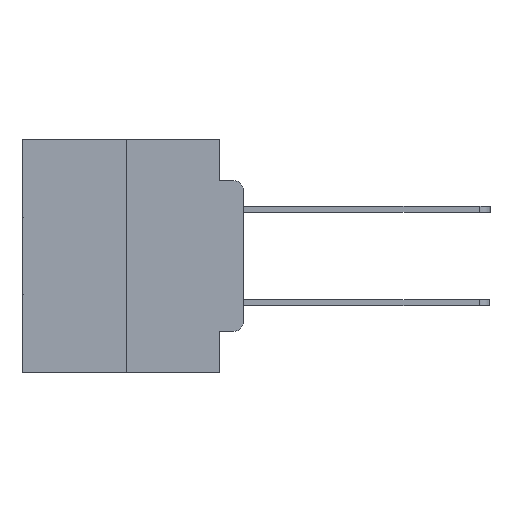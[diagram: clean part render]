
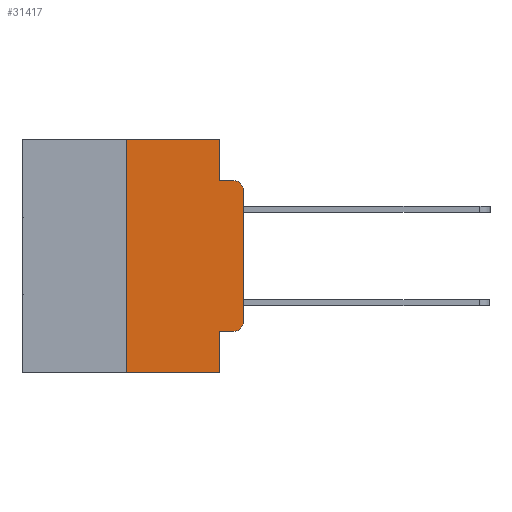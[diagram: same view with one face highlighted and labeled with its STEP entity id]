
A CAD part, left-side view. The second image highlights one B-rep face of the part: STEP entity #31417.
In plain terms, the highlighted planar face has unit normal (-1, 0, 0).
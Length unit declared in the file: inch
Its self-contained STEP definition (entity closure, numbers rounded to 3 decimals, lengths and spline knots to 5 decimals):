
#404 = VERTEX_POINT ( 'NONE', #24986 ) ;
#2196 = DIRECTION ( 'NONE',  ( -1., 0., 0. ) ) ;
#2727 = CARTESIAN_POINT ( 'NONE',  ( 0., 0.051, -0.5 ) ) ;
#2791 = ORIENTED_EDGE ( 'NONE', *, *, #20344, .T. ) ;
#3180 = CARTESIAN_POINT ( 'NONE',  ( 0., 0.02, -0.1085 ) ) ;
#3460 = DIRECTION ( 'NONE',  ( 0., 0., -1. ) ) ;
#4398 = CARTESIAN_POINT ( 'NONE',  ( 0., 0.051, -0.4115 ) ) ;
#4464 = VECTOR ( 'NONE', #26174, 39.37008 ) ;
#4697 = CARTESIAN_POINT ( 'NONE',  ( 0., 0., 0. ) ) ;
#5798 = DIRECTION ( 'NONE',  ( 0., 0., -1. ) ) ;
#6577 = LINE ( 'NONE', #20827, #12320 ) ;
#6727 = EDGE_CURVE ( 'NONE', #28806, #22925, #30735, .T. ) ;
#6857 = DIRECTION ( 'NONE',  ( 0., 0., -1. ) ) ;
#6976 = VERTEX_POINT ( 'NONE', #17495 ) ;
#7261 = CARTESIAN_POINT ( 'NONE',  ( 0., 0., -0.3915 ) ) ;
#7346 = EDGE_CURVE ( 'NONE', #23276, #28806, #10422, .T. ) ;
#7831 = DIRECTION ( 'NONE',  ( 0., -1., 0. ) ) ;
#8003 = ORIENTED_EDGE ( 'NONE', *, *, #7346, .F. ) ;
#8252 = ORIENTED_EDGE ( 'NONE', *, *, #17773, .T. ) ;
#8449 = PLANE ( 'NONE',  #17743 ) ;
#9687 = DIRECTION ( 'NONE',  ( 0., 0., 1. ) ) ;
#9902 = CARTESIAN_POINT ( 'NONE',  ( 0., 0.051, -0.0885 ) ) ;
#10422 = LINE ( 'NONE', #25810, #29554 ) ;
#10742 = CIRCLE ( 'NONE', #16157, 0.02 ) ;
#10863 = CARTESIAN_POINT ( 'NONE',  ( 0., 0.473, 0. ) ) ;
#10952 = VERTEX_POINT ( 'NONE', #24384 ) ;
#11019 = LINE ( 'NONE', #4398, #4464 ) ;
#11647 = DIRECTION ( 'NONE',  ( 0., -1., 0. ) ) ;
#11868 = CARTESIAN_POINT ( 'NONE',  ( 0., 0.25, 0. ) ) ;
#12257 = EDGE_CURVE ( 'NONE', #22925, #14688, #27369, .T. ) ;
#12268 = DIRECTION ( 'NONE',  ( 0., 0., -1. ) ) ;
#12320 = VECTOR ( 'NONE', #23184, 39.37008 ) ;
#12950 = VECTOR ( 'NONE', #6857, 39.37008 ) ;
#13734 = EDGE_CURVE ( 'NONE', #23276, #25001, #6577, .T. ) ;
#13882 = EDGE_CURVE ( 'NONE', #14688, #6976, #27634, .T. ) ;
#13956 = AXIS2_PLACEMENT_3D ( 'NONE', #3180, #20356, #5798 ) ;
#14688 = VERTEX_POINT ( 'NONE', #9902 ) ;
#16157 = AXIS2_PLACEMENT_3D ( 'NONE', #17071, #2196, #19486 ) ;
#17071 = CARTESIAN_POINT ( 'NONE',  ( 0., 0.02, -0.3915 ) ) ;
#17495 = CARTESIAN_POINT ( 'NONE',  ( 0., 0.02, -0.0885 ) ) ;
#17743 = AXIS2_PLACEMENT_3D ( 'NONE', #10863, #18246, #3460 ) ;
#17773 = EDGE_CURVE ( 'NONE', #10952, #21394, #10742, .T. ) ;
#18129 = VECTOR ( 'NONE', #7831, 39.37008 ) ;
#18246 = DIRECTION ( 'NONE',  ( 1., 0., 0. ) ) ;
#18682 = ORIENTED_EDGE ( 'NONE', *, *, #27275, .F. ) ;
#18913 = FACE_OUTER_BOUND ( 'NONE', #22596, .T. ) ;
#19021 = ORIENTED_EDGE ( 'NONE', *, *, #13882, .F. ) ;
#19377 = EDGE_CURVE ( 'NONE', #404, #10952, #11019, .T. ) ;
#19486 = DIRECTION ( 'NONE',  ( 0., 0., -1. ) ) ;
#20344 = EDGE_CURVE ( 'NONE', #30033, #6976, #26011, .T. ) ;
#20356 = DIRECTION ( 'NONE',  ( -1., 0., 0. ) ) ;
#20592 = VECTOR ( 'NONE', #11647, 39.37008 ) ;
#20827 = CARTESIAN_POINT ( 'NONE',  ( 0., 0.473, -0.5 ) ) ;
#20966 = DIRECTION ( 'NONE',  ( 0., 0., 1. ) ) ;
#21048 = VECTOR ( 'NONE', #12268, 39.37008 ) ;
#21216 = CARTESIAN_POINT ( 'NONE',  ( 0., 0.051, -0.0885 ) ) ;
#21394 = VERTEX_POINT ( 'NONE', #7261 ) ;
#21785 = CARTESIAN_POINT ( 'NONE',  ( 0., 0., -0.1085 ) ) ;
#21818 = CARTESIAN_POINT ( 'NONE',  ( 0., 0.051, 0. ) ) ;
#22596 = EDGE_LOOP ( 'NONE', ( #26373, #2791, #19021, #28256, #31254, #8003, #28653, #18682, #27934, #8252 ) ) ;
#22925 = VERTEX_POINT ( 'NONE', #28086 ) ;
#23092 = LINE ( 'NONE', #4697, #28686 ) ;
#23184 = DIRECTION ( 'NONE',  ( 0., -1., 0. ) ) ;
#23276 = VERTEX_POINT ( 'NONE', #26933 ) ;
#24384 = CARTESIAN_POINT ( 'NONE',  ( 0., 0.02, -0.4115 ) ) ;
#24926 = LINE ( 'NONE', #31002, #12950 ) ;
#24986 = CARTESIAN_POINT ( 'NONE',  ( 0., 0.051, -0.4115 ) ) ;
#25001 = VERTEX_POINT ( 'NONE', #2727 ) ;
#25810 = CARTESIAN_POINT ( 'NONE',  ( 0., 0.25, 0. ) ) ;
#26011 = CIRCLE ( 'NONE', #13956, 0.02 ) ;
#26174 = DIRECTION ( 'NONE',  ( 0., -1., 0. ) ) ;
#26373 = ORIENTED_EDGE ( 'NONE', *, *, #26684, .T. ) ;
#26684 = EDGE_CURVE ( 'NONE', #21394, #30033, #23092, .T. ) ;
#26933 = CARTESIAN_POINT ( 'NONE',  ( 0., 0.25, -0.5 ) ) ;
#27045 = CARTESIAN_POINT ( 'NONE',  ( 0., 0.473, 0. ) ) ;
#27275 = EDGE_CURVE ( 'NONE', #404, #25001, #24926, .T. ) ;
#27369 = LINE ( 'NONE', #21818, #21048 ) ;
#27634 = LINE ( 'NONE', #21216, #20592 ) ;
#27934 = ORIENTED_EDGE ( 'NONE', *, *, #19377, .T. ) ;
#28086 = CARTESIAN_POINT ( 'NONE',  ( 0., 0.051, 0. ) ) ;
#28256 = ORIENTED_EDGE ( 'NONE', *, *, #12257, .F. ) ;
#28653 = ORIENTED_EDGE ( 'NONE', *, *, #13734, .T. ) ;
#28686 = VECTOR ( 'NONE', #9687, 39.37008 ) ;
#28806 = VERTEX_POINT ( 'NONE', #11868 ) ;
#29554 = VECTOR ( 'NONE', #20966, 39.37008 ) ;
#30033 = VERTEX_POINT ( 'NONE', #21785 ) ;
#30735 = LINE ( 'NONE', #27045, #18129 ) ;
#31002 = CARTESIAN_POINT ( 'NONE',  ( 0., 0.051, 0. ) ) ;
#31254 = ORIENTED_EDGE ( 'NONE', *, *, #6727, .F. ) ;
#31417 = ADVANCED_FACE ( 'NONE', ( #18913 ), #8449, .F. ) ;
